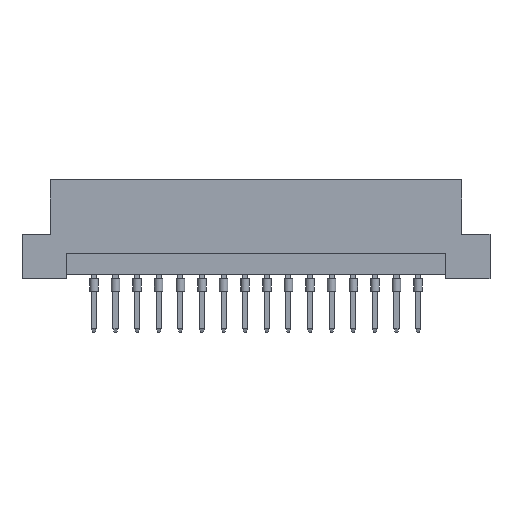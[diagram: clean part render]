
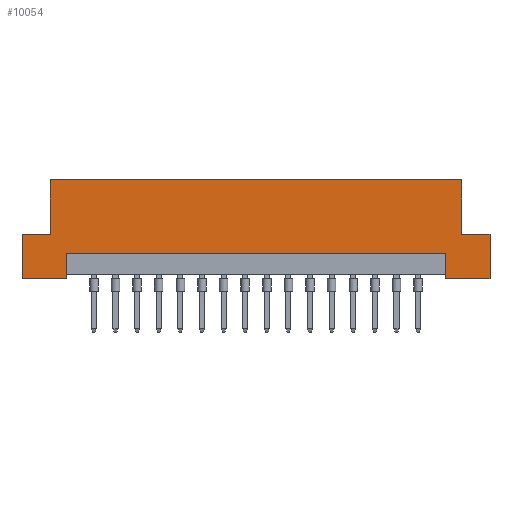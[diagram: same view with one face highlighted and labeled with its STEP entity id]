
A CAD part, front view. The second image highlights one B-rep face of the part: STEP entity #10054.
In plain terms, the highlighted planar face has unit normal (0, -1, 0).
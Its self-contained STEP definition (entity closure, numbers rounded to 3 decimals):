
#24 = LINE ( 'NONE', #9832, #7948 ) ;
#70 = CARTESIAN_POINT ( 'NONE',  ( -27.5, 0., 0. ) ) ;
#290 = VECTOR ( 'NONE', #7001, 1000. ) ;
#339 = CARTESIAN_POINT ( 'NONE',  ( -27.5, 0., 0. ) ) ;
#525 = DIRECTION ( 'NONE',  ( 0., 0., 1. ) ) ;
#594 = CARTESIAN_POINT ( 'NONE',  ( -27.5, 0., 0. ) ) ;
#754 = CARTESIAN_POINT ( 'NONE',  ( -27.5, 0., 11.6 ) ) ;
#810 = DIRECTION ( 'NONE',  ( 1., 0., 0. ) ) ;
#814 = VECTOR ( 'NONE', #810, 1000. ) ;
#844 = CARTESIAN_POINT ( 'NONE',  ( 22.3, 0., 2.9 ) ) ;
#1310 = EDGE_CURVE ( 'NONE', #4260, #10479, #6184, .T. ) ;
#1335 = VECTOR ( 'NONE', #3298, 1000. ) ;
#1452 = CARTESIAN_POINT ( 'NONE',  ( 27.5, 0., 0. ) ) ;
#1556 = EDGE_CURVE ( 'NONE', #3930, #5912, #4197, .T. ) ;
#1589 = DIRECTION ( 'NONE',  ( 0., 0., -1. ) ) ;
#1610 = EDGE_CURVE ( 'NONE', #10479, #10309, #5117, .T. ) ;
#1633 = EDGE_CURVE ( 'NONE', #4511, #9809, #8373, .T. ) ;
#1767 = VERTEX_POINT ( 'NONE', #6871 ) ;
#1931 = ORIENTED_EDGE ( 'NONE', *, *, #1633, .F. ) ;
#1957 = ORIENTED_EDGE ( 'NONE', *, *, #5044, .F. ) ;
#1973 = LINE ( 'NONE', #2643, #6676 ) ;
#2065 = ORIENTED_EDGE ( 'NONE', *, *, #9202, .F. ) ;
#2107 = DIRECTION ( 'NONE',  ( 1., 0., 0. ) ) ;
#2298 = VERTEX_POINT ( 'NONE', #844 ) ;
#2606 = LINE ( 'NONE', #754, #7166 ) ;
#2634 = EDGE_CURVE ( 'NONE', #2298, #9809, #8653, .T. ) ;
#2643 = CARTESIAN_POINT ( 'NONE',  ( 24.2, 0., 5.2 ) ) ;
#3227 = CARTESIAN_POINT ( 'NONE',  ( -27.5, 0., 11.6 ) ) ;
#3278 = CARTESIAN_POINT ( 'NONE',  ( -27.5, 0., 5.2 ) ) ;
#3298 = DIRECTION ( 'NONE',  ( -1., 0., 0. ) ) ;
#3362 = VECTOR ( 'NONE', #8789, 1000. ) ;
#3502 = CARTESIAN_POINT ( 'NONE',  ( -24.2, 0., 5.2 ) ) ;
#3764 = CARTESIAN_POINT ( 'NONE',  ( 22.3, 0., 0. ) ) ;
#3766 = CARTESIAN_POINT ( 'NONE',  ( 24.2, 0., 5.2 ) ) ;
#3780 = CARTESIAN_POINT ( 'NONE',  ( 22.3, 0., 2.9 ) ) ;
#3835 = ORIENTED_EDGE ( 'NONE', *, *, #9210, .F. ) ;
#3930 = VERTEX_POINT ( 'NONE', #3766 ) ;
#4097 = VERTEX_POINT ( 'NONE', #339 ) ;
#4113 = LINE ( 'NONE', #70, #5566 ) ;
#4148 = DIRECTION ( 'NONE',  ( 0., 0., 1. ) ) ;
#4197 = LINE ( 'NONE', #7459, #814 ) ;
#4200 = ORIENTED_EDGE ( 'NONE', *, *, #1556, .F. ) ;
#4260 = VERTEX_POINT ( 'NONE', #3278 ) ;
#4368 = CARTESIAN_POINT ( 'NONE',  ( -22.3, 0., 0. ) ) ;
#4485 = CARTESIAN_POINT ( 'NONE',  ( 22.3, 0., 0.5 ) ) ;
#4511 = VERTEX_POINT ( 'NONE', #9514 ) ;
#4605 = ORIENTED_EDGE ( 'NONE', *, *, #1610, .F. ) ;
#4649 = DIRECTION ( 'NONE',  ( 0., 0., -1. ) ) ;
#4784 = VECTOR ( 'NONE', #2107, 1000. ) ;
#5044 = EDGE_CURVE ( 'NONE', #4097, #4260, #8704, .T. ) ;
#5117 = LINE ( 'NONE', #3502, #6124 ) ;
#5235 = EDGE_CURVE ( 'NONE', #10309, #8511, #2606, .T. ) ;
#5535 = LINE ( 'NONE', #3780, #3362 ) ;
#5566 = VECTOR ( 'NONE', #5776, 1000. ) ;
#5644 = DIRECTION ( 'NONE',  ( 0., 0., -1. ) ) ;
#5699 = CARTESIAN_POINT ( 'NONE',  ( -27.5, 0., 0. ) ) ;
#5776 = DIRECTION ( 'NONE',  ( -1., 0., 0. ) ) ;
#5912 = VERTEX_POINT ( 'NONE', #6757 ) ;
#6124 = VECTOR ( 'NONE', #4148, 1000. ) ;
#6184 = LINE ( 'NONE', #9445, #4784 ) ;
#6247 = ORIENTED_EDGE ( 'NONE', *, *, #9460, .F. ) ;
#6294 = VERTEX_POINT ( 'NONE', #4368 ) ;
#6588 = EDGE_LOOP ( 'NONE', ( #7018, #9936, #1931, #6247, #4200, #9858, #10109, #4605, #6752, #1957, #3835, #2065 ) ) ;
#6602 = CARTESIAN_POINT ( 'NONE',  ( 24.2, 0., 11.6 ) ) ;
#6676 = VECTOR ( 'NONE', #7602, 1000. ) ;
#6752 = ORIENTED_EDGE ( 'NONE', *, *, #1310, .F. ) ;
#6757 = CARTESIAN_POINT ( 'NONE',  ( 27.5, 0., 5.2 ) ) ;
#6790 = VECTOR ( 'NONE', #4649, 1000. ) ;
#6871 = CARTESIAN_POINT ( 'NONE',  ( -22.3, 0., 2.9 ) ) ;
#7001 = DIRECTION ( 'NONE',  ( 0., 0., 1. ) ) ;
#7018 = ORIENTED_EDGE ( 'NONE', *, *, #8286, .F. ) ;
#7166 = VECTOR ( 'NONE', #7311, 1000. ) ;
#7188 = EDGE_CURVE ( 'NONE', #3930, #8511, #1973, .T. ) ;
#7311 = DIRECTION ( 'NONE',  ( 1., 0., 0. ) ) ;
#7459 = CARTESIAN_POINT ( 'NONE',  ( 27.5, 0., 5.2 ) ) ;
#7590 = CARTESIAN_POINT ( 'NONE',  ( -24.2, 0., 11.6 ) ) ;
#7602 = DIRECTION ( 'NONE',  ( 0., 0., 1. ) ) ;
#7874 = DIRECTION ( 'NONE',  ( 0., 1., 0. ) ) ;
#7948 = VECTOR ( 'NONE', #1589, 1000. ) ;
#8046 = LINE ( 'NONE', #1452, #10174 ) ;
#8069 = CARTESIAN_POINT ( 'NONE',  ( -24.2, 0., 5.2 ) ) ;
#8286 = EDGE_CURVE ( 'NONE', #2298, #1767, #5535, .T. ) ;
#8373 = LINE ( 'NONE', #5699, #1335 ) ;
#8511 = VERTEX_POINT ( 'NONE', #6602 ) ;
#8653 = LINE ( 'NONE', #4485, #6790 ) ;
#8704 = LINE ( 'NONE', #594, #290 ) ;
#8789 = DIRECTION ( 'NONE',  ( -1., 0., 0. ) ) ;
#8894 = PLANE ( 'NONE',  #9201 ) ;
#9201 = AXIS2_PLACEMENT_3D ( 'NONE', #3227, #7874, #525 ) ;
#9202 = EDGE_CURVE ( 'NONE', #1767, #6294, #24, .T. ) ;
#9210 = EDGE_CURVE ( 'NONE', #6294, #4097, #4113, .T. ) ;
#9445 = CARTESIAN_POINT ( 'NONE',  ( -27.5, 0., 5.2 ) ) ;
#9460 = EDGE_CURVE ( 'NONE', #5912, #4511, #8046, .T. ) ;
#9514 = CARTESIAN_POINT ( 'NONE',  ( 27.5, 0., 0. ) ) ;
#9809 = VERTEX_POINT ( 'NONE', #3764 ) ;
#9832 = CARTESIAN_POINT ( 'NONE',  ( -22.3, 0., 0.5 ) ) ;
#9858 = ORIENTED_EDGE ( 'NONE', *, *, #7188, .T. ) ;
#9936 = ORIENTED_EDGE ( 'NONE', *, *, #2634, .T. ) ;
#10054 = ADVANCED_FACE ( 'NONE', ( #10502 ), #8894, .F. ) ;
#10109 = ORIENTED_EDGE ( 'NONE', *, *, #5235, .F. ) ;
#10174 = VECTOR ( 'NONE', #5644, 1000. ) ;
#10309 = VERTEX_POINT ( 'NONE', #7590 ) ;
#10479 = VERTEX_POINT ( 'NONE', #8069 ) ;
#10502 = FACE_OUTER_BOUND ( 'NONE', #6588, .T. ) ;
